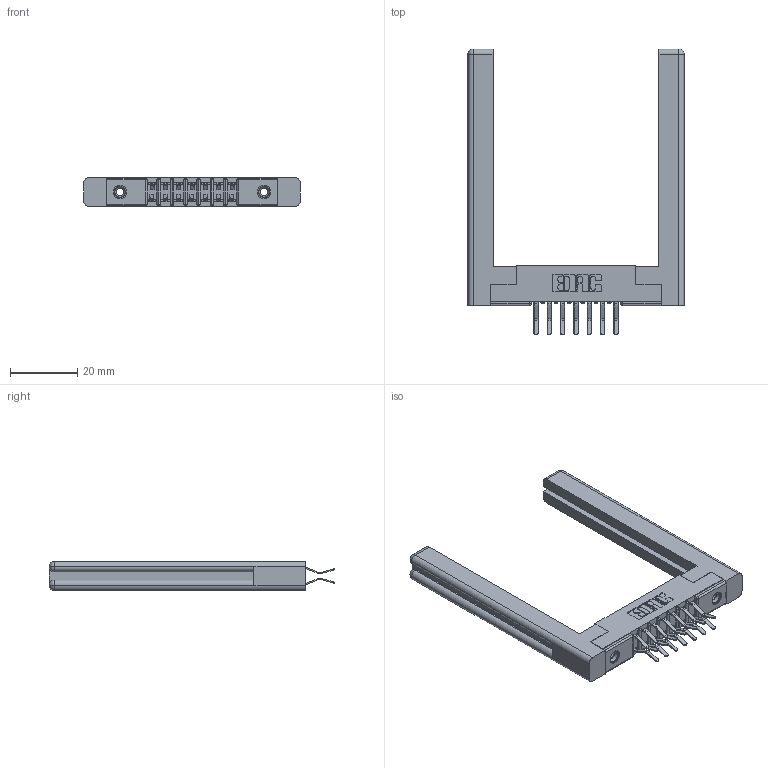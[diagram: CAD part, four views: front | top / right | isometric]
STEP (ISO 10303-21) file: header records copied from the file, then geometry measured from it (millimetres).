
FILE_DESCRIPTION (( 'STEP AP203' ), '1' );
FILE_NAME ('357-014-460-258.STEP', '2020-10-02T18:32:19', ( '' ), ( '' ), 'SwSTEP 2.0', 'SolidWorks 2020', '' );
FILE_SCHEMA (( 'CONFIG_CONTROL_DESIGN' ));
Length unit declared in the file: inch
Products named in the file (5): 357-014-460-258; 307-290-001_560; 307 Part_.156 Dia Mounting Holes; 345-250-001_345-250-001-102; 307-220-058
Assembly tree (19 placements, depth 2):
  357-014-460-258
    307 Part_.156 Dia Mounting Holes
    307-290-001_560  x14
    307-220-058  x2
    345-250-001_345-250-001-102  x2
Bounding box: 64.36 x 85.04 x 8.71 mm (x, y, z)
Volume: 11915.8 mm3; surface area: 11883 mm2
Topology: 19 solids, 19 shells, 968 faces, 2665 edges, 1722 vertices
Faces by surface type: plane 616, cylinder 312, sphere 16, torus 12, cone 12
Entity records: 13277 total; most frequent: CARTESIAN_POINT 2202, DIRECTION 2130, ORIENTED_EDGE 2120, EDGE_CURVE 1060, VECTOR 794, LINE 794, VERTEX_POINT 686, AXIS2_PLACEMENT_3D 668
